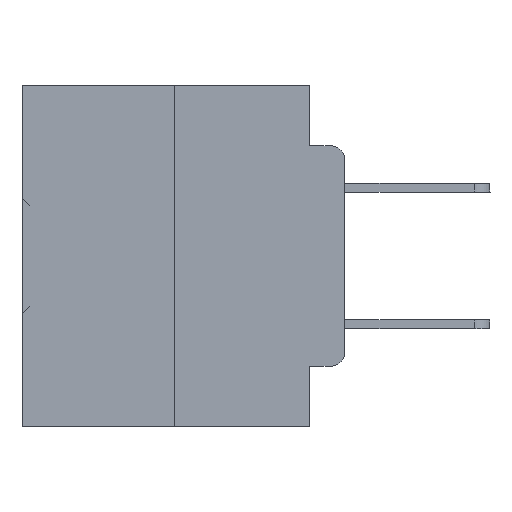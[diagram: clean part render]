
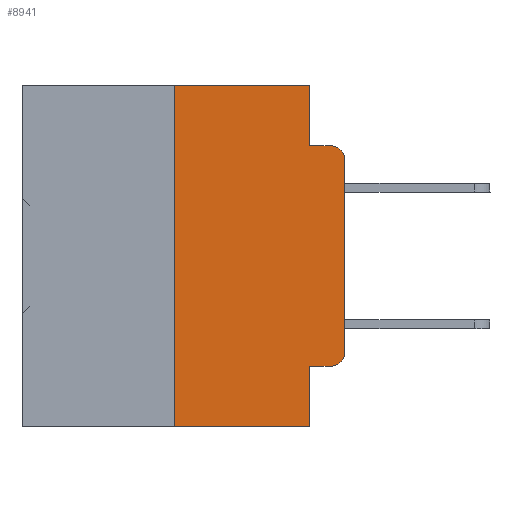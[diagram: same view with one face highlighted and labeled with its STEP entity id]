
A CAD part, left-side view. The second image highlights one B-rep face of the part: STEP entity #8941.
In plain terms, the highlighted planar face has unit normal (-1, 0, 0).
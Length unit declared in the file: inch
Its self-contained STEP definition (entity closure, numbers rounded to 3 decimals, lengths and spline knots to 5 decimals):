
#97 = ORIENTED_EDGE ( 'NONE', *, *, #26660, .F. ) ;
#245 = LINE ( 'NONE', #12364, #36196 ) ;
#909 = AXIS2_PLACEMENT_3D ( 'NONE', #33994, #16277, #34600 ) ;
#3231 = VERTEX_POINT ( 'NONE', #28225 ) ;
#3241 = CARTESIAN_POINT ( 'NONE',  ( 0., 0.02, -0.0885 ) ) ;
#3305 = VERTEX_POINT ( 'NONE', #21671 ) ;
#4017 = AXIS2_PLACEMENT_3D ( 'NONE', #15969, #27305, #27500 ) ;
#4131 = VERTEX_POINT ( 'NONE', #18917 ) ;
#4157 = CARTESIAN_POINT ( 'NONE',  ( 0., 0.473, 0. ) ) ;
#6220 = ORIENTED_EDGE ( 'NONE', *, *, #32256, .T. ) ;
#6363 = CARTESIAN_POINT ( 'NONE',  ( 0., 0.25, -0.5 ) ) ;
#6953 = LINE ( 'NONE', #37351, #16400 ) ;
#7279 = CIRCLE ( 'NONE', #909, 0.02 ) ;
#7583 = ORIENTED_EDGE ( 'NONE', *, *, #34114, .F. ) ;
#8036 = VERTEX_POINT ( 'NONE', #30703 ) ;
#8920 = DIRECTION ( 'NONE',  ( 0., -1., 0. ) ) ;
#8941 = ADVANCED_FACE ( 'NONE', ( #15489 ), #36965, .F. ) ;
#9199 = CARTESIAN_POINT ( 'NONE',  ( 0., 0.051, -0.4115 ) ) ;
#9212 = EDGE_CURVE ( 'NONE', #32591, #8036, #9627, .T. ) ;
#9627 = LINE ( 'NONE', #18543, #37305 ) ;
#10872 = VECTOR ( 'NONE', #19487, 39.37008 ) ;
#12364 = CARTESIAN_POINT ( 'NONE',  ( 0., 0., 0. ) ) ;
#12428 = CARTESIAN_POINT ( 'NONE',  ( 0., 0.051, -0.0885 ) ) ;
#12581 = LINE ( 'NONE', #22116, #19690 ) ;
#12773 = VERTEX_POINT ( 'NONE', #31594 ) ;
#13069 = CARTESIAN_POINT ( 'NONE',  ( 0., 0.051, 0. ) ) ;
#13981 = CARTESIAN_POINT ( 'NONE',  ( 0., 0.051, -0.4115 ) ) ;
#15107 = CARTESIAN_POINT ( 'NONE',  ( 0., 0., -0.3915 ) ) ;
#15220 = DIRECTION ( 'NONE',  ( 0., -1., 0. ) ) ;
#15439 = CIRCLE ( 'NONE', #4017, 0.02 ) ;
#15489 = FACE_OUTER_BOUND ( 'NONE', #24551, .T. ) ;
#15540 = LINE ( 'NONE', #9199, #15939 ) ;
#15939 = VECTOR ( 'NONE', #26896, 39.37008 ) ;
#15969 = CARTESIAN_POINT ( 'NONE',  ( 0., 0.02, -0.1085 ) ) ;
#16277 = DIRECTION ( 'NONE',  ( -1., 0., 0. ) ) ;
#16400 = VECTOR ( 'NONE', #19040, 39.37008 ) ;
#18506 = VECTOR ( 'NONE', #15220, 39.37008 ) ;
#18543 = CARTESIAN_POINT ( 'NONE',  ( 0., 0.473, -0.5 ) ) ;
#18552 = EDGE_CURVE ( 'NONE', #25356, #4131, #15540, .T. ) ;
#18917 = CARTESIAN_POINT ( 'NONE',  ( 0., 0.02, -0.4115 ) ) ;
#19040 = DIRECTION ( 'NONE',  ( 0., 0., 1. ) ) ;
#19487 = DIRECTION ( 'NONE',  ( 0., 0., -1. ) ) ;
#19690 = VECTOR ( 'NONE', #24912, 39.37008 ) ;
#19998 = VERTEX_POINT ( 'NONE', #15107 ) ;
#21456 = ORIENTED_EDGE ( 'NONE', *, *, #9212, .T. ) ;
#21465 = EDGE_CURVE ( 'NONE', #4131, #19998, #7279, .T. ) ;
#21484 = DIRECTION ( 'NONE',  ( 0., 0., 1. ) ) ;
#21631 = ORIENTED_EDGE ( 'NONE', *, *, #35694, .F. ) ;
#21671 = CARTESIAN_POINT ( 'NONE',  ( 0., 0.25, 0. ) ) ;
#22116 = CARTESIAN_POINT ( 'NONE',  ( 0., 0.473, 0. ) ) ;
#23708 = ORIENTED_EDGE ( 'NONE', *, *, #34616, .F. ) ;
#24551 = EDGE_LOOP ( 'NONE', ( #6220, #27095, #21631, #7583, #23708, #27205, #21456, #97, #34350, #28193 ) ) ;
#24912 = DIRECTION ( 'NONE',  ( 0., -1., 0. ) ) ;
#25356 = VERTEX_POINT ( 'NONE', #13981 ) ;
#26660 = EDGE_CURVE ( 'NONE', #25356, #8036, #36587, .T. ) ;
#26896 = DIRECTION ( 'NONE',  ( 0., -1., 0. ) ) ;
#27095 = ORIENTED_EDGE ( 'NONE', *, *, #37353, .T. ) ;
#27205 = ORIENTED_EDGE ( 'NONE', *, *, #31493, .F. ) ;
#27305 = DIRECTION ( 'NONE',  ( -1., 0., 0. ) ) ;
#27500 = DIRECTION ( 'NONE',  ( 0., 0., -1. ) ) ;
#28193 = ORIENTED_EDGE ( 'NONE', *, *, #21465, .T. ) ;
#28225 = CARTESIAN_POINT ( 'NONE',  ( 0., 0., -0.1085 ) ) ;
#28486 = VECTOR ( 'NONE', #29857, 39.37008 ) ;
#29857 = DIRECTION ( 'NONE',  ( 0., 0., -1. ) ) ;
#30227 = CARTESIAN_POINT ( 'NONE',  ( 0., 0.051, 0. ) ) ;
#30703 = CARTESIAN_POINT ( 'NONE',  ( 0., 0.051, -0.5 ) ) ;
#31390 = DIRECTION ( 'NONE',  ( 0., 0., -1. ) ) ;
#31426 = VERTEX_POINT ( 'NONE', #13069 ) ;
#31493 = EDGE_CURVE ( 'NONE', #32591, #3305, #6953, .T. ) ;
#31594 = CARTESIAN_POINT ( 'NONE',  ( 0., 0.051, -0.0885 ) ) ;
#32256 = EDGE_CURVE ( 'NONE', #19998, #3231, #245, .T. ) ;
#32591 = VERTEX_POINT ( 'NONE', #6363 ) ;
#33711 = LINE ( 'NONE', #12428, #18506 ) ;
#33929 = VERTEX_POINT ( 'NONE', #3241 ) ;
#33994 = CARTESIAN_POINT ( 'NONE',  ( 0., 0.02, -0.3915 ) ) ;
#34114 = EDGE_CURVE ( 'NONE', #31426, #12773, #37020, .T. ) ;
#34177 = DIRECTION ( 'NONE',  ( 1., 0., 0. ) ) ;
#34240 = CARTESIAN_POINT ( 'NONE',  ( 0., 0.051, 0. ) ) ;
#34350 = ORIENTED_EDGE ( 'NONE', *, *, #18552, .T. ) ;
#34600 = DIRECTION ( 'NONE',  ( 0., 0., -1. ) ) ;
#34616 = EDGE_CURVE ( 'NONE', #3305, #31426, #12581, .T. ) ;
#35694 = EDGE_CURVE ( 'NONE', #12773, #33929, #33711, .T. ) ;
#36196 = VECTOR ( 'NONE', #21484, 39.37008 ) ;
#36587 = LINE ( 'NONE', #30227, #28486 ) ;
#36965 = PLANE ( 'NONE',  #38603 ) ;
#37020 = LINE ( 'NONE', #34240, #10872 ) ;
#37305 = VECTOR ( 'NONE', #8920, 39.37008 ) ;
#37351 = CARTESIAN_POINT ( 'NONE',  ( 0., 0.25, 0. ) ) ;
#37353 = EDGE_CURVE ( 'NONE', #3231, #33929, #15439, .T. ) ;
#38603 = AXIS2_PLACEMENT_3D ( 'NONE', #4157, #34177, #31390 ) ;
